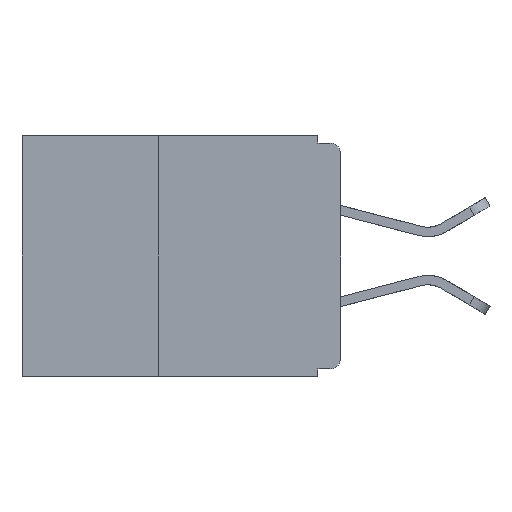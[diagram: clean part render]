
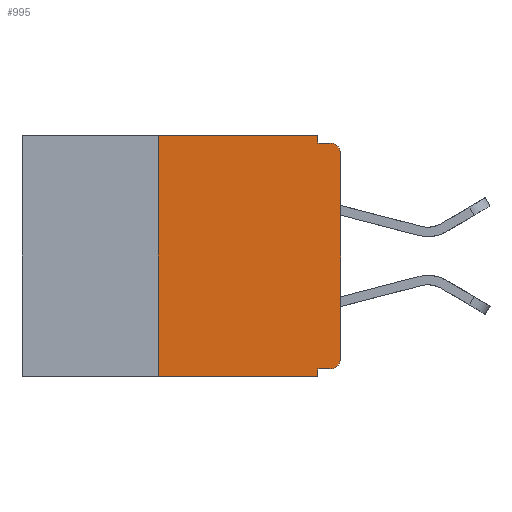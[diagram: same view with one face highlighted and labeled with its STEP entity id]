
A CAD part, left-side view. The second image highlights one B-rep face of the part: STEP entity #995.
In plain terms, the highlighted planar face has unit normal (-1, 0, 0).
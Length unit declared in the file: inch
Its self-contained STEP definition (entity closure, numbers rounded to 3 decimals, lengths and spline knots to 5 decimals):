
#276 = VERTEX_POINT ( 'NONE', #22585 ) ;
#350 = EDGE_CURVE ( 'NONE', #23472, #7813, #26321, .T. ) ;
#995 = ADVANCED_FACE ( 'NONE', ( #27531 ), #21891, .F. ) ;
#1435 = ORIENTED_EDGE ( 'NONE', *, *, #12983, .T. ) ;
#1486 = DIRECTION ( 'NONE',  ( 0., 0., -1. ) ) ;
#1974 = LINE ( 'NONE', #16966, #23267 ) ;
#2188 = VECTOR ( 'NONE', #11949, 39.37008 ) ;
#2758 = ORIENTED_EDGE ( 'NONE', *, *, #28947, .T. ) ;
#3422 = EDGE_CURVE ( 'NONE', #23471, #33345, #16376, .T. ) ;
#4064 = VECTOR ( 'NONE', #1486, 39.37008 ) ;
#4078 = ORIENTED_EDGE ( 'NONE', *, *, #27555, .F. ) ;
#4717 = EDGE_CURVE ( 'NONE', #11827, #10580, #26036, .T. ) ;
#5286 = CARTESIAN_POINT ( 'NONE',  ( 0., 0.437, -0.33 ) ) ;
#6209 = DIRECTION ( 'NONE',  ( -1., 0., 0. ) ) ;
#6266 = AXIS2_PLACEMENT_3D ( 'NONE', #11102, #30246, #13958 ) ;
#6798 = CARTESIAN_POINT ( 'NONE',  ( 0., 0.25, -0.33 ) ) ;
#7573 = ORIENTED_EDGE ( 'NONE', *, *, #12349, .F. ) ;
#7813 = VERTEX_POINT ( 'NONE', #8184 ) ;
#8175 = VECTOR ( 'NONE', #35322, 39.37008 ) ;
#8184 = CARTESIAN_POINT ( 'NONE',  ( 0., 0.015, -0.01 ) ) ;
#8596 = DIRECTION ( 'NONE',  ( 0., 1., 0. ) ) ;
#8891 = VECTOR ( 'NONE', #18507, 39.37008 ) ;
#9130 = DIRECTION ( 'NONE',  ( 0., 0., -1. ) ) ;
#9355 = LINE ( 'NONE', #22906, #15094 ) ;
#10294 = EDGE_CURVE ( 'NONE', #14503, #276, #15706, .T. ) ;
#10580 = VERTEX_POINT ( 'NONE', #14934 ) ;
#10958 = EDGE_CURVE ( 'NONE', #16714, #12045, #1974, .T. ) ;
#11102 = CARTESIAN_POINT ( 'NONE',  ( 0., 0.015, -0.305 ) ) ;
#11827 = VERTEX_POINT ( 'NONE', #6798 ) ;
#11949 = DIRECTION ( 'NONE',  ( 0., -1., 0. ) ) ;
#12045 = VERTEX_POINT ( 'NONE', #35124 ) ;
#12202 = CARTESIAN_POINT ( 'NONE',  ( 0., 0.031, -0.01 ) ) ;
#12349 = EDGE_CURVE ( 'NONE', #12045, #10580, #9355, .T. ) ;
#12642 = DIRECTION ( 'NONE',  ( 0., -1., 0. ) ) ;
#12983 = EDGE_CURVE ( 'NONE', #276, #7813, #26514, .T. ) ;
#13373 = CARTESIAN_POINT ( 'NONE',  ( 0., 0.25, -0.33 ) ) ;
#13604 = CARTESIAN_POINT ( 'NONE',  ( 0., 0., 0. ) ) ;
#13958 = DIRECTION ( 'NONE',  ( 0., 0., -1. ) ) ;
#14108 = CARTESIAN_POINT ( 'NONE',  ( 0., 0.015, -0.32 ) ) ;
#14231 = ORIENTED_EDGE ( 'NONE', *, *, #4717, .T. ) ;
#14503 = VERTEX_POINT ( 'NONE', #25090 ) ;
#14888 = CARTESIAN_POINT ( 'NONE',  ( 0., 0.437, 0. ) ) ;
#14934 = CARTESIAN_POINT ( 'NONE',  ( 0., 0.031, -0.33 ) ) ;
#15094 = VECTOR ( 'NONE', #9130, 39.37008 ) ;
#15160 = AXIS2_PLACEMENT_3D ( 'NONE', #22859, #6209, #25584 ) ;
#15706 = LINE ( 'NONE', #13604, #8175 ) ;
#15985 = LINE ( 'NONE', #13373, #29531 ) ;
#16187 = DIRECTION ( 'NONE',  ( 0., 0., 1. ) ) ;
#16267 = AXIS2_PLACEMENT_3D ( 'NONE', #23294, #21875, #21249 ) ;
#16376 = LINE ( 'NONE', #14888, #8891 ) ;
#16714 = VERTEX_POINT ( 'NONE', #14108 ) ;
#16737 = CIRCLE ( 'NONE', #6266, 0.015 ) ;
#16966 = CARTESIAN_POINT ( 'NONE',  ( 0., 0., -0.32 ) ) ;
#18135 = ORIENTED_EDGE ( 'NONE', *, *, #350, .F. ) ;
#18507 = DIRECTION ( 'NONE',  ( 0., -1., 0. ) ) ;
#19282 = EDGE_LOOP ( 'NONE', ( #28268, #1435, #18135, #4078, #34124, #20711, #14231, #7573, #29555, #2758 ) ) ;
#19826 = LINE ( 'NONE', #34403, #4064 ) ;
#20711 = ORIENTED_EDGE ( 'NONE', *, *, #34735, .F. ) ;
#21249 = DIRECTION ( 'NONE',  ( 0., 0., -1. ) ) ;
#21875 = DIRECTION ( 'NONE',  ( 1., 0., 0. ) ) ;
#21891 = PLANE ( 'NONE',  #16267 ) ;
#22585 = CARTESIAN_POINT ( 'NONE',  ( 0., 0., -0.025 ) ) ;
#22859 = CARTESIAN_POINT ( 'NONE',  ( 0., 0.015, -0.025 ) ) ;
#22906 = CARTESIAN_POINT ( 'NONE',  ( 0., 0.031, -0.33 ) ) ;
#23267 = VECTOR ( 'NONE', #8596, 39.37008 ) ;
#23294 = CARTESIAN_POINT ( 'NONE',  ( 0., 0.437, 0. ) ) ;
#23471 = VERTEX_POINT ( 'NONE', #28563 ) ;
#23472 = VERTEX_POINT ( 'NONE', #12202 ) ;
#24568 = CARTESIAN_POINT ( 'NONE',  ( 0., 0.031, 0. ) ) ;
#25090 = CARTESIAN_POINT ( 'NONE',  ( 0., 0., -0.305 ) ) ;
#25440 = VECTOR ( 'NONE', #12642, 39.37008 ) ;
#25584 = DIRECTION ( 'NONE',  ( 0., 0., -1. ) ) ;
#26036 = LINE ( 'NONE', #5286, #2188 ) ;
#26321 = LINE ( 'NONE', #35126, #25440 ) ;
#26514 = CIRCLE ( 'NONE', #15160, 0.015 ) ;
#27531 = FACE_OUTER_BOUND ( 'NONE', #19282, .T. ) ;
#27555 = EDGE_CURVE ( 'NONE', #33345, #23472, #19826, .T. ) ;
#28268 = ORIENTED_EDGE ( 'NONE', *, *, #10294, .T. ) ;
#28563 = CARTESIAN_POINT ( 'NONE',  ( 0., 0.25, 0. ) ) ;
#28947 = EDGE_CURVE ( 'NONE', #16714, #14503, #16737, .T. ) ;
#29531 = VECTOR ( 'NONE', #16187, 39.37008 ) ;
#29555 = ORIENTED_EDGE ( 'NONE', *, *, #10958, .F. ) ;
#30246 = DIRECTION ( 'NONE',  ( -1., 0., 0. ) ) ;
#33345 = VERTEX_POINT ( 'NONE', #24568 ) ;
#34124 = ORIENTED_EDGE ( 'NONE', *, *, #3422, .F. ) ;
#34403 = CARTESIAN_POINT ( 'NONE',  ( 0., 0.031, 0. ) ) ;
#34735 = EDGE_CURVE ( 'NONE', #11827, #23471, #15985, .T. ) ;
#35124 = CARTESIAN_POINT ( 'NONE',  ( 0., 0.031, -0.32 ) ) ;
#35126 = CARTESIAN_POINT ( 'NONE',  ( 0., 0., -0.01 ) ) ;
#35322 = DIRECTION ( 'NONE',  ( 0., 0., 1. ) ) ;
